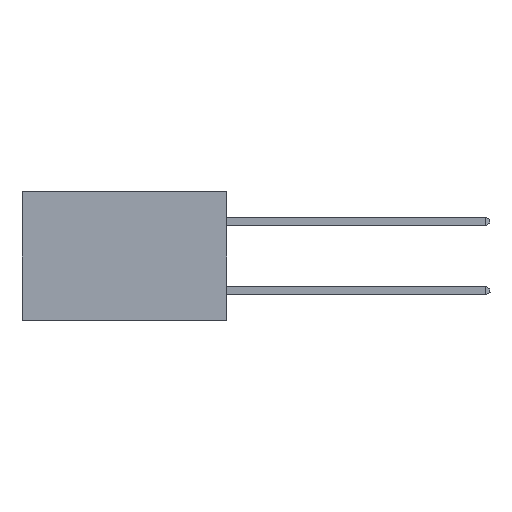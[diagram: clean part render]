
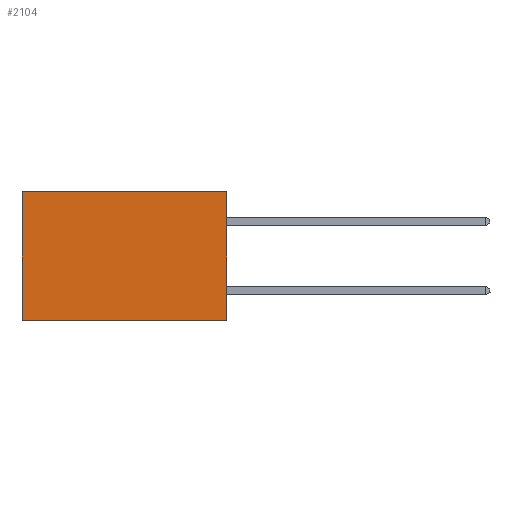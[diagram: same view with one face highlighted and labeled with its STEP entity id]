
A CAD part, left-side view. The second image highlights one B-rep face of the part: STEP entity #2104.
In plain terms, the highlighted planar face has unit normal (-1, 0, 0).
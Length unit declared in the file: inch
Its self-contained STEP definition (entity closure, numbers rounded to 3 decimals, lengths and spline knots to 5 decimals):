
#101 = CARTESIAN_POINT ( 'NONE',  ( 0.277, 0., 0. ) ) ;
#1192 = LINE ( 'NONE', #22598, #7719 ) ;
#1990 = DIRECTION ( 'NONE',  ( 0., 0., -1. ) ) ;
#2104 = ADVANCED_FACE ( 'NONE', ( #7019 ), #31466, .F. ) ;
#2252 = LINE ( 'NONE', #31878, #22189 ) ;
#2282 = ORIENTED_EDGE ( 'NONE', *, *, #18242, .T. ) ;
#2955 = DIRECTION ( 'NONE',  ( 0., 1., 0. ) ) ;
#3560 = VECTOR ( 'NONE', #6430, 39.37008 ) ;
#3584 = CARTESIAN_POINT ( 'NONE',  ( 0.277, 0., -0.37 ) ) ;
#4052 = VERTEX_POINT ( 'NONE', #24313 ) ;
#4422 = LINE ( 'NONE', #19847, #3560 ) ;
#5869 = EDGE_CURVE ( 'NONE', #4052, #6490, #2252, .T. ) ;
#5963 = DIRECTION ( 'NONE',  ( 0., 0., -1. ) ) ;
#6430 = DIRECTION ( 'NONE',  ( 0., 0., -1. ) ) ;
#6490 = VERTEX_POINT ( 'NONE', #19472 ) ;
#6843 = VERTEX_POINT ( 'NONE', #7902 ) ;
#7019 = FACE_OUTER_BOUND ( 'NONE', #17860, .T. ) ;
#7719 = VECTOR ( 'NONE', #9253, 39.37008 ) ;
#7902 = CARTESIAN_POINT ( 'NONE',  ( 0.277, 0.59, 0. ) ) ;
#9253 = DIRECTION ( 'NONE',  ( 0., 1., 0. ) ) ;
#11197 = ORIENTED_EDGE ( 'NONE', *, *, #21245, .F. ) ;
#12493 = EDGE_CURVE ( 'NONE', #6843, #6490, #22830, .T. ) ;
#15708 = VECTOR ( 'NONE', #5963, 39.37008 ) ;
#16139 = ORIENTED_EDGE ( 'NONE', *, *, #12493, .T. ) ;
#16598 = AXIS2_PLACEMENT_3D ( 'NONE', #3584, #31958, #1990 ) ;
#17860 = EDGE_LOOP ( 'NONE', ( #16139, #20385, #11197, #2282 ) ) ;
#18242 = EDGE_CURVE ( 'NONE', #19355, #6843, #1192, .T. ) ;
#19355 = VERTEX_POINT ( 'NONE', #101 ) ;
#19472 = CARTESIAN_POINT ( 'NONE',  ( 0.277, 0.59, -0.37 ) ) ;
#19847 = CARTESIAN_POINT ( 'NONE',  ( 0.277, 0., -0.37 ) ) ;
#20385 = ORIENTED_EDGE ( 'NONE', *, *, #5869, .F. ) ;
#21245 = EDGE_CURVE ( 'NONE', #19355, #4052, #4422, .T. ) ;
#22189 = VECTOR ( 'NONE', #2955, 39.37008 ) ;
#22598 = CARTESIAN_POINT ( 'NONE',  ( 0.277, 0., 0. ) ) ;
#22830 = LINE ( 'NONE', #24775, #15708 ) ;
#24313 = CARTESIAN_POINT ( 'NONE',  ( 0.277, 0., -0.37 ) ) ;
#24775 = CARTESIAN_POINT ( 'NONE',  ( 0.277, 0.59, -0.37 ) ) ;
#31466 = PLANE ( 'NONE',  #16598 ) ;
#31878 = CARTESIAN_POINT ( 'NONE',  ( 0.277, 0., -0.37 ) ) ;
#31958 = DIRECTION ( 'NONE',  ( 1., 0., 0. ) ) ;
